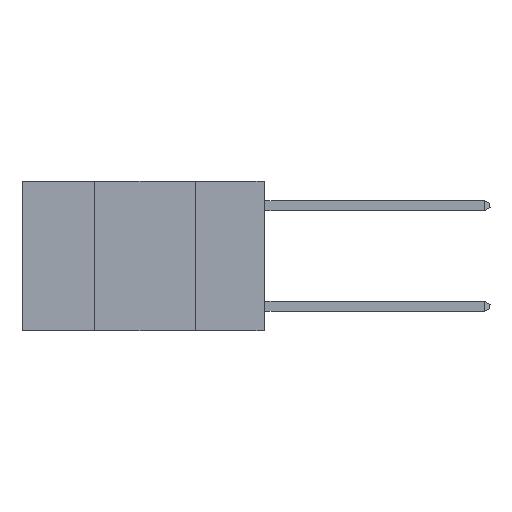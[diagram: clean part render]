
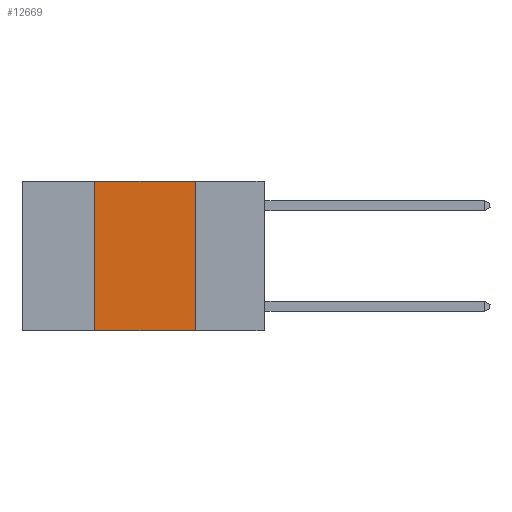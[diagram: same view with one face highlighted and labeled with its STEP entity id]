
A CAD part, left-side view. The second image highlights one B-rep face of the part: STEP entity #12669.
In plain terms, the highlighted planar face has unit normal (-1, 0, 0).
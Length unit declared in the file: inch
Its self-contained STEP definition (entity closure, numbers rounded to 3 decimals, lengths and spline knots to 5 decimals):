
#86 = DIRECTION ( 'NONE',  ( 1., 0., 0. ) ) ;
#1560 = CARTESIAN_POINT ( 'NONE',  ( 0., 0.6, 0. ) ) ;
#3272 = VECTOR ( 'NONE', #4503, 39.37008 ) ;
#3522 = DIRECTION ( 'NONE',  ( 0., 0., -1. ) ) ;
#3639 = EDGE_CURVE ( 'NONE', #18649, #10953, #14879, .T. ) ;
#3927 = VERTEX_POINT ( 'NONE', #4698 ) ;
#4503 = DIRECTION ( 'NONE',  ( 0., 0., 1. ) ) ;
#4698 = CARTESIAN_POINT ( 'NONE',  ( 0., 0.42, -0.37 ) ) ;
#5468 = EDGE_CURVE ( 'NONE', #3927, #18949, #13938, .T. ) ;
#5646 = CARTESIAN_POINT ( 'NONE',  ( 0., 0.17, -0.37 ) ) ;
#7108 = DIRECTION ( 'NONE',  ( 0., 0., -1. ) ) ;
#10190 = DIRECTION ( 'NONE',  ( 0., -1., 0. ) ) ;
#10313 = EDGE_CURVE ( 'NONE', #18949, #18649, #22059, .T. ) ;
#10953 = VERTEX_POINT ( 'NONE', #5646 ) ;
#12309 = ORIENTED_EDGE ( 'NONE', *, *, #10313, .F. ) ;
#12638 = VECTOR ( 'NONE', #3522, 39.37008 ) ;
#12669 = ADVANCED_FACE ( 'NONE', ( #13701 ), #27503, .F. ) ;
#13636 = VECTOR ( 'NONE', #19805, 39.37008 ) ;
#13701 = FACE_OUTER_BOUND ( 'NONE', #15482, .T. ) ;
#13870 = ORIENTED_EDGE ( 'NONE', *, *, #25425, .T. ) ;
#13938 = LINE ( 'NONE', #23076, #3272 ) ;
#14879 = LINE ( 'NONE', #26290, #12638 ) ;
#15482 = EDGE_LOOP ( 'NONE', ( #28185, #12309, #18212, #13870 ) ) ;
#17232 = LINE ( 'NONE', #26386, #17308 ) ;
#17308 = VECTOR ( 'NONE', #10190, 39.37008 ) ;
#18212 = ORIENTED_EDGE ( 'NONE', *, *, #5468, .F. ) ;
#18649 = VERTEX_POINT ( 'NONE', #27488 ) ;
#18949 = VERTEX_POINT ( 'NONE', #26423 ) ;
#19805 = DIRECTION ( 'NONE',  ( 0., -1., 0. ) ) ;
#22059 = LINE ( 'NONE', #1560, #13636 ) ;
#23076 = CARTESIAN_POINT ( 'NONE',  ( 0., 0.42, 0. ) ) ;
#25425 = EDGE_CURVE ( 'NONE', #3927, #10953, #17232, .T. ) ;
#26290 = CARTESIAN_POINT ( 'NONE',  ( 0., 0.17, 0. ) ) ;
#26386 = CARTESIAN_POINT ( 'NONE',  ( 0., 0.6, -0.37 ) ) ;
#26423 = CARTESIAN_POINT ( 'NONE',  ( 0., 0.42, 0. ) ) ;
#27004 = AXIS2_PLACEMENT_3D ( 'NONE', #27660, #86, #7108 ) ;
#27488 = CARTESIAN_POINT ( 'NONE',  ( 0., 0.17, 0. ) ) ;
#27503 = PLANE ( 'NONE',  #27004 ) ;
#27660 = CARTESIAN_POINT ( 'NONE',  ( 0., 0.6, 0. ) ) ;
#28185 = ORIENTED_EDGE ( 'NONE', *, *, #3639, .F. ) ;
